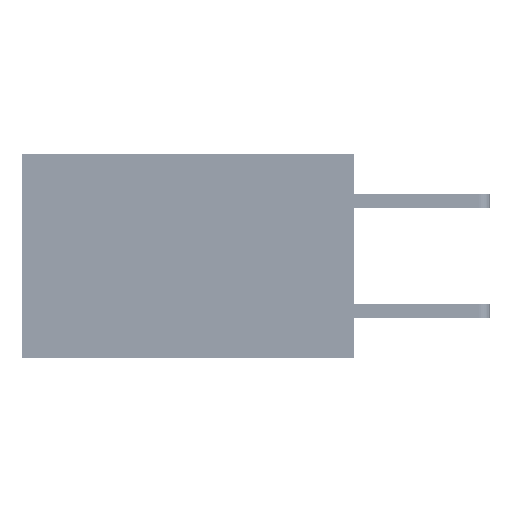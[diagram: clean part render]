
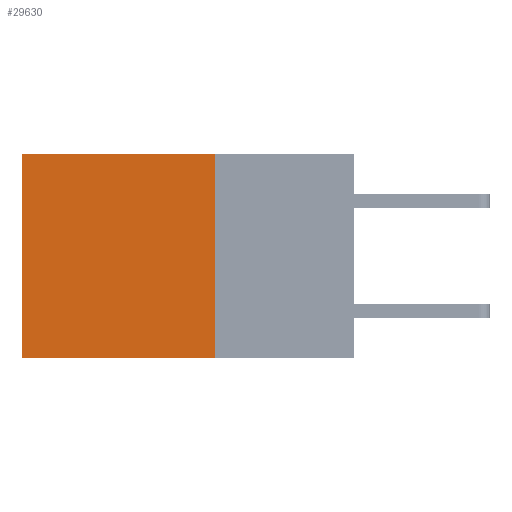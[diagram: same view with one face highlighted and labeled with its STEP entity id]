
A CAD part, left-side view. The second image highlights one B-rep face of the part: STEP entity #29630.
In plain terms, the highlighted planar face has unit normal (-1, 0, 0).
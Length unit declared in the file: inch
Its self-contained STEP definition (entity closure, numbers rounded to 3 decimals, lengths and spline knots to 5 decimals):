
#120 = DIRECTION ( 'NONE',  ( 0., 0., -1. ) ) ;
#606 = VECTOR ( 'NONE', #44407, 39.37008 ) ;
#679 = CARTESIAN_POINT ( 'NONE',  ( 0.2875, 0.6, 0. ) ) ;
#734 = VERTEX_POINT ( 'NONE', #40712 ) ;
#1547 = DIRECTION ( 'NONE',  ( 0., 0., -1. ) ) ;
#4334 = VECTOR ( 'NONE', #1547, 39.37008 ) ;
#4418 = VECTOR ( 'NONE', #42915, 39.37008 ) ;
#4852 = CARTESIAN_POINT ( 'NONE',  ( 0.2875, 0.6, 0. ) ) ;
#6108 = ORIENTED_EDGE ( 'NONE', *, *, #29221, .F. ) ;
#8903 = DIRECTION ( 'NONE',  ( 0., 1., 0. ) ) ;
#9824 = LINE ( 'NONE', #33848, #606 ) ;
#14320 = EDGE_LOOP ( 'NONE', ( #31091, #32371, #6108, #26416 ) ) ;
#15387 = LINE ( 'NONE', #29340, #25421 ) ;
#15440 = VERTEX_POINT ( 'NONE', #38017 ) ;
#15824 = LINE ( 'NONE', #4852, #4418 ) ;
#20794 = DIRECTION ( 'NONE',  ( 1., 0., 0. ) ) ;
#23635 = LINE ( 'NONE', #42760, #4334 ) ;
#25421 = VECTOR ( 'NONE', #8903, 39.37008 ) ;
#26416 = ORIENTED_EDGE ( 'NONE', *, *, #31453, .T. ) ;
#27399 = CARTESIAN_POINT ( 'NONE',  ( 0.2875, 0.25, 0. ) ) ;
#28324 = AXIS2_PLACEMENT_3D ( 'NONE', #27399, #20794, #120 ) ;
#29221 = EDGE_CURVE ( 'NONE', #15440, #734, #23635, .T. ) ;
#29340 = CARTESIAN_POINT ( 'NONE',  ( 0.2875, 0.25, -0.37 ) ) ;
#29630 = ADVANCED_FACE ( 'NONE', ( #42589 ), #41329, .F. ) ;
#29976 = EDGE_CURVE ( 'NONE', #734, #40206, #15387, .T. ) ;
#31091 = ORIENTED_EDGE ( 'NONE', *, *, #31161, .T. ) ;
#31161 = EDGE_CURVE ( 'NONE', #41606, #40206, #15824, .T. ) ;
#31453 = EDGE_CURVE ( 'NONE', #15440, #41606, #9824, .T. ) ;
#32371 = ORIENTED_EDGE ( 'NONE', *, *, #29976, .F. ) ;
#33848 = CARTESIAN_POINT ( 'NONE',  ( 0.2875, 0.25, 0. ) ) ;
#38017 = CARTESIAN_POINT ( 'NONE',  ( 0.2875, 0.25, 0. ) ) ;
#38891 = CARTESIAN_POINT ( 'NONE',  ( 0.2875, 0.6, -0.37 ) ) ;
#40206 = VERTEX_POINT ( 'NONE', #38891 ) ;
#40712 = CARTESIAN_POINT ( 'NONE',  ( 0.2875, 0.25, -0.37 ) ) ;
#41329 = PLANE ( 'NONE',  #28324 ) ;
#41606 = VERTEX_POINT ( 'NONE', #679 ) ;
#42589 = FACE_OUTER_BOUND ( 'NONE', #14320, .T. ) ;
#42760 = CARTESIAN_POINT ( 'NONE',  ( 0.2875, 0.25, 0. ) ) ;
#42915 = DIRECTION ( 'NONE',  ( 0., 0., -1. ) ) ;
#44407 = DIRECTION ( 'NONE',  ( 0., 1., 0. ) ) ;
